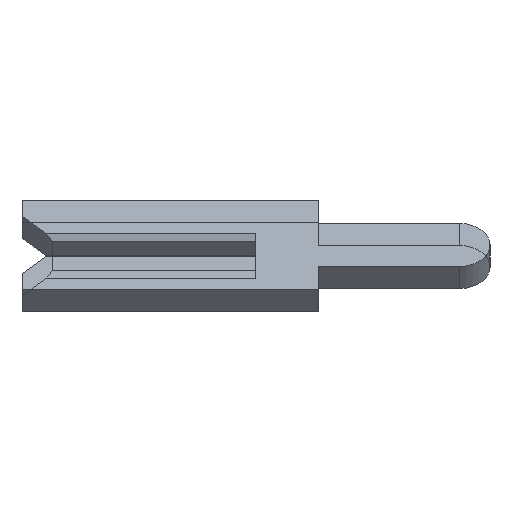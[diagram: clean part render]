
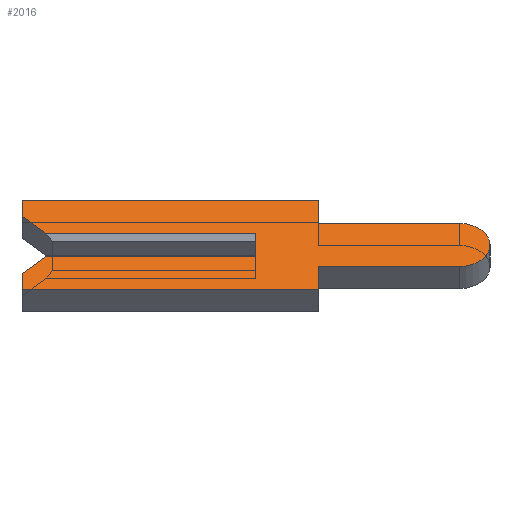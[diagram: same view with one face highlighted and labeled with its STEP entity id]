
A CAD part, left-side view. The second image highlights one B-rep face of the part: STEP entity #2016.
In plain terms, the highlighted face is planar.
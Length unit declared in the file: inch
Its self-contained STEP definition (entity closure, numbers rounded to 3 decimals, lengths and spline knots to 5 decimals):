
#21 = LINE ( 'NONE', #1997, #1801 ) ;
#34 = CARTESIAN_POINT ( 'NONE',  ( -0.01, -0.04, 0.04 ) ) ;
#65 = DIRECTION ( 'NONE',  ( 0., 0., -1. ) ) ;
#169 = ORIENTED_EDGE ( 'NONE', *, *, #2221, .T. ) ;
#194 = LINE ( 'NONE', #864, #2916 ) ;
#206 = EDGE_CURVE ( 'NONE', #1041, #1707, #2693, .T. ) ;
#210 = VERTEX_POINT ( 'NONE', #1656 ) ;
#231 = VERTEX_POINT ( 'NONE', #600 ) ;
#245 = LINE ( 'NONE', #836, #1690 ) ;
#288 = CARTESIAN_POINT ( 'NONE',  ( -0.01, -0.04, -0.0195 ) ) ;
#385 = EDGE_CURVE ( 'NONE', #3107, #1041, #768, .T. ) ;
#401 = VERTEX_POINT ( 'NONE', #633 ) ;
#476 = CARTESIAN_POINT ( 'NONE',  ( -0.01, 0.15, 0.01 ) ) ;
#521 = DIRECTION ( 'NONE',  ( 0., -1., 0. ) ) ;
#562 = CARTESIAN_POINT ( 'NONE',  ( -0.01, -0.04, 0.04 ) ) ;
#600 = CARTESIAN_POINT ( 'NONE',  ( -0.01, 0., 0.01 ) ) ;
#633 = CARTESIAN_POINT ( 'NONE',  ( -0.01, 0.15, -0.026 ) ) ;
#751 = VECTOR ( 'NONE', #3441, 39.37008 ) ;
#768 = CIRCLE ( 'NONE', #2665, 0.0195 ) ;
#807 = VECTOR ( 'NONE', #2170, 39.37008 ) ;
#836 = CARTESIAN_POINT ( 'NONE',  ( -0.01, -0.1305, -0.01 ) ) ;
#864 = CARTESIAN_POINT ( 'NONE',  ( -0.01, 0.15, 0.04 ) ) ;
#899 = VERTEX_POINT ( 'NONE', #1427 ) ;
#967 = DIRECTION ( 'NONE',  ( 0., 1., 0. ) ) ;
#1021 = VECTOR ( 'NONE', #1932, 39.37008 ) ;
#1041 = VERTEX_POINT ( 'NONE', #3556 ) ;
#1139 = VECTOR ( 'NONE', #4378, 39.37008 ) ;
#1179 = VERTEX_POINT ( 'NONE', #3573 ) ;
#1219 = VECTOR ( 'NONE', #967, 39.37008 ) ;
#1257 = LINE ( 'NONE', #1859, #2572 ) ;
#1362 = FACE_OUTER_BOUND ( 'NONE', #1926, .T. ) ;
#1427 = CARTESIAN_POINT ( 'NONE',  ( -0.01, 0.134, -0.01 ) ) ;
#1517 = CARTESIAN_POINT ( 'NONE',  ( -0.01, -0.04, -0.0195 ) ) ;
#1551 = CARTESIAN_POINT ( 'NONE',  ( -0.01, 0.1305, 0.0065 ) ) ;
#1587 = LINE ( 'NONE', #4331, #3594 ) ;
#1594 = DIRECTION ( 'NONE',  ( 0., -1., 0. ) ) ;
#1631 = EDGE_CURVE ( 'NONE', #1707, #3453, #3139, .T. ) ;
#1640 = VERTEX_POINT ( 'NONE', #34 ) ;
#1652 = ORIENTED_EDGE ( 'NONE', *, *, #2194, .F. ) ;
#1656 = CARTESIAN_POINT ( 'NONE',  ( -0.01, 0., -0.01 ) ) ;
#1690 = VECTOR ( 'NONE', #1594, 39.37008 ) ;
#1707 = VERTEX_POINT ( 'NONE', #1517 ) ;
#1801 = VECTOR ( 'NONE', #3074, 39.37008 ) ;
#1830 = VERTEX_POINT ( 'NONE', #4363 ) ;
#1831 = EDGE_CURVE ( 'NONE', #2755, #1830, #1257, .T. ) ;
#1846 = PLANE ( 'NONE',  #3305 ) ;
#1859 = CARTESIAN_POINT ( 'NONE',  ( -0.01, 0.15, 0.026 ) ) ;
#1890 = DIRECTION ( 'NONE',  ( 0., -0.707, 0.707 ) ) ;
#1926 = EDGE_LOOP ( 'NONE', ( #169, #1652, #2876, #2609, #1937, #4294, #4058, #3494, #2887, #2205, #3938, #4112, #2615, #2335 ) ) ;
#1932 = DIRECTION ( 'NONE',  ( 0., 0.707, 0.707 ) ) ;
#1937 = ORIENTED_EDGE ( 'NONE', *, *, #3419, .F. ) ;
#1997 = CARTESIAN_POINT ( 'NONE',  ( -0.01, 0.15, -0.04 ) ) ;
#2012 = VECTOR ( 'NONE', #521, 39.37008 ) ;
#2016 = ADVANCED_FACE ( 'NONE', ( #1362 ), #1846, .F. ) ;
#2058 = EDGE_CURVE ( 'NONE', #401, #899, #1587, .T. ) ;
#2170 = DIRECTION ( 'NONE',  ( 0., 0., -1. ) ) ;
#2187 = LINE ( 'NONE', #4076, #1139 ) ;
#2192 = DIRECTION ( 'NONE',  ( 1., 0., 0. ) ) ;
#2194 = EDGE_CURVE ( 'NONE', #210, #231, #2187, .T. ) ;
#2205 = ORIENTED_EDGE ( 'NONE', *, *, #2944, .F. ) ;
#2221 = EDGE_CURVE ( 'NONE', #3623, #231, #4084, .T. ) ;
#2300 = CARTESIAN_POINT ( 'NONE',  ( -0.01, -0.1305, 0.0195 ) ) ;
#2310 = EDGE_CURVE ( 'NONE', #1830, #1640, #194, .T. ) ;
#2335 = ORIENTED_EDGE ( 'NONE', *, *, #2336, .F. ) ;
#2336 = EDGE_CURVE ( 'NONE', #3623, #2755, #2857, .T. ) ;
#2572 = VECTOR ( 'NONE', #2914, 39.37008 ) ;
#2590 = DIRECTION ( 'NONE',  ( 0., -1., 0. ) ) ;
#2609 = ORIENTED_EDGE ( 'NONE', *, *, #2058, .F. ) ;
#2615 = ORIENTED_EDGE ( 'NONE', *, *, #1831, .F. ) ;
#2637 = CARTESIAN_POINT ( 'NONE',  ( -0.01, -0.04, 0.0195 ) ) ;
#2665 = AXIS2_PLACEMENT_3D ( 'NONE', #4243, #3888, #3165 ) ;
#2693 = LINE ( 'NONE', #288, #1219 ) ;
#2709 = CARTESIAN_POINT ( 'NONE',  ( -0.01, 0.15, -0.026 ) ) ;
#2734 = LINE ( 'NONE', #2637, #2012 ) ;
#2755 = VERTEX_POINT ( 'NONE', #3724 ) ;
#2857 = LINE ( 'NONE', #1551, #1021 ) ;
#2876 = ORIENTED_EDGE ( 'NONE', *, *, #3056, .F. ) ;
#2887 = ORIENTED_EDGE ( 'NONE', *, *, #385, .F. ) ;
#2914 = DIRECTION ( 'NONE',  ( 0., 0., 1. ) ) ;
#2916 = VECTOR ( 'NONE', #2590, 39.37008 ) ;
#2930 = CARTESIAN_POINT ( 'NONE',  ( -0.01, -0.1305, 0. ) ) ;
#2944 = EDGE_CURVE ( 'NONE', #3082, #3107, #2734, .T. ) ;
#3056 = EDGE_CURVE ( 'NONE', #899, #210, #245, .T. ) ;
#3074 = DIRECTION ( 'NONE',  ( 0., 1., 0. ) ) ;
#3082 = VERTEX_POINT ( 'NONE', #3347 ) ;
#3107 = VERTEX_POINT ( 'NONE', #2300 ) ;
#3131 = VECTOR ( 'NONE', #3408, 39.37008 ) ;
#3139 = LINE ( 'NONE', #3288, #807 ) ;
#3165 = DIRECTION ( 'NONE',  ( 0., 0., -1. ) ) ;
#3288 = CARTESIAN_POINT ( 'NONE',  ( -0.01, -0.04, -0.04 ) ) ;
#3305 = AXIS2_PLACEMENT_3D ( 'NONE', #2930, #2192, #65 ) ;
#3334 = EDGE_CURVE ( 'NONE', #3453, #1179, #21, .T. ) ;
#3347 = CARTESIAN_POINT ( 'NONE',  ( -0.01, -0.04, 0.0195 ) ) ;
#3408 = DIRECTION ( 'NONE',  ( 0., 0., -1. ) ) ;
#3419 = EDGE_CURVE ( 'NONE', #1179, #401, #3644, .T. ) ;
#3441 = DIRECTION ( 'NONE',  ( 0., 0., 1. ) ) ;
#3453 = VERTEX_POINT ( 'NONE', #4132 ) ;
#3494 = ORIENTED_EDGE ( 'NONE', *, *, #206, .F. ) ;
#3556 = CARTESIAN_POINT ( 'NONE',  ( -0.01, -0.1305, -0.0195 ) ) ;
#3573 = CARTESIAN_POINT ( 'NONE',  ( -0.01, 0.15, -0.04 ) ) ;
#3594 = VECTOR ( 'NONE', #1890, 39.37008 ) ;
#3623 = VERTEX_POINT ( 'NONE', #3787 ) ;
#3644 = LINE ( 'NONE', #2709, #751 ) ;
#3706 = DIRECTION ( 'NONE',  ( 0., -1., 0. ) ) ;
#3724 = CARTESIAN_POINT ( 'NONE',  ( -0.01, 0.15, 0.026 ) ) ;
#3761 = VECTOR ( 'NONE', #3706, 39.37008 ) ;
#3787 = CARTESIAN_POINT ( 'NONE',  ( -0.01, 0.134, 0.01 ) ) ;
#3888 = DIRECTION ( 'NONE',  ( 1., 0., 0. ) ) ;
#3938 = ORIENTED_EDGE ( 'NONE', *, *, #4436, .F. ) ;
#4058 = ORIENTED_EDGE ( 'NONE', *, *, #1631, .F. ) ;
#4076 = CARTESIAN_POINT ( 'NONE',  ( -0.01, 0., 0.0065 ) ) ;
#4084 = LINE ( 'NONE', #476, #3761 ) ;
#4112 = ORIENTED_EDGE ( 'NONE', *, *, #2310, .F. ) ;
#4132 = CARTESIAN_POINT ( 'NONE',  ( -0.01, -0.04, -0.04 ) ) ;
#4243 = CARTESIAN_POINT ( 'NONE',  ( -0.01, -0.1305, 0. ) ) ;
#4294 = ORIENTED_EDGE ( 'NONE', *, *, #3334, .F. ) ;
#4331 = CARTESIAN_POINT ( 'NONE',  ( -0.01, 0.1305, -0.0065 ) ) ;
#4363 = CARTESIAN_POINT ( 'NONE',  ( -0.01, 0.15, 0.04 ) ) ;
#4367 = LINE ( 'NONE', #562, #3131 ) ;
#4378 = DIRECTION ( 'NONE',  ( 0., 0., 1. ) ) ;
#4436 = EDGE_CURVE ( 'NONE', #1640, #3082, #4367, .T. ) ;
